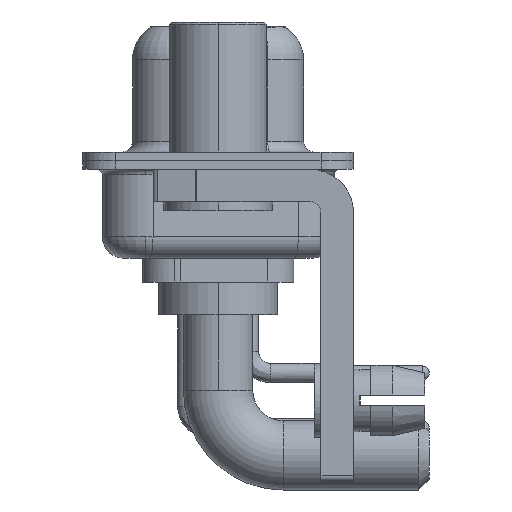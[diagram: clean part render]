
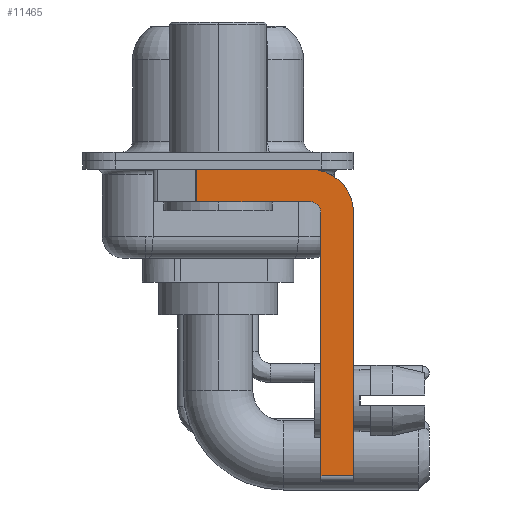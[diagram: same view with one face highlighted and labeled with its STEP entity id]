
A CAD part, left-side view. The second image highlights one B-rep face of the part: STEP entity #11465.
In plain terms, the highlighted planar face has unit normal (-1, 0, 0).
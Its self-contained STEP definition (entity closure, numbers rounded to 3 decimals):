
#335 = LINE ( 'NONE', #8071, #6720 ) ;
#677 = DIRECTION ( 'NONE',  ( -1., 0., 0. ) ) ;
#1410 = LINE ( 'NONE', #19088, #17224 ) ;
#1963 = CARTESIAN_POINT ( 'NONE',  ( -2.9, -4.25, -1.9 ) ) ;
#2416 = LINE ( 'NONE', #6575, #20677 ) ;
#2481 = VERTEX_POINT ( 'NONE', #11726 ) ;
#2768 = VERTEX_POINT ( 'NONE', #10321 ) ;
#3099 = DIRECTION ( 'NONE',  ( 0., 0., 1. ) ) ;
#3500 = LINE ( 'NONE', #6896, #24793 ) ;
#3735 = VERTEX_POINT ( 'NONE', #5189 ) ;
#4128 = EDGE_CURVE ( 'NONE', #4290, #12373, #3500, .T. ) ;
#4290 = VERTEX_POINT ( 'NONE', #1963 ) ;
#4563 = EDGE_CURVE ( 'NONE', #2481, #3735, #11192, .T. ) ;
#5189 = CARTESIAN_POINT ( 'NONE',  ( -2.9, -6.25, -2.4 ) ) ;
#6121 = ORIENTED_EDGE ( 'NONE', *, *, #11451, .F. ) ;
#6187 = DIRECTION ( 'NONE',  ( 0., 0., -1. ) ) ;
#6575 = CARTESIAN_POINT ( 'NONE',  ( -2.9, 0.978, -1.9 ) ) ;
#6720 = VECTOR ( 'NONE', #6187, 1000. ) ;
#6869 = DIRECTION ( 'NONE',  ( 1., 0., 0. ) ) ;
#6896 = CARTESIAN_POINT ( 'NONE',  ( -2.9, -4.25, -1.9 ) ) ;
#7363 = CARTESIAN_POINT ( 'NONE',  ( -2.9, 3., -0.4 ) ) ;
#7474 = CARTESIAN_POINT ( 'NONE',  ( -2.9, -4.75, -2.4 ) ) ;
#7487 = DIRECTION ( 'NONE',  ( 1., 0., 0. ) ) ;
#7610 = DIRECTION ( 'NONE',  ( 0., -1., 0. ) ) ;
#7772 = EDGE_CURVE ( 'NONE', #17053, #24008, #14337, .T. ) ;
#8071 = CARTESIAN_POINT ( 'NONE',  ( -2.9, -6.25, -2.4 ) ) ;
#8200 = VECTOR ( 'NONE', #12199, 1000. ) ;
#8413 = CARTESIAN_POINT ( 'NONE',  ( -2.9, -4.25, -2.4 ) ) ;
#8598 = DIRECTION ( 'NONE',  ( 0., 0., -1. ) ) ;
#8790 = ORIENTED_EDGE ( 'NONE', *, *, #18653, .F. ) ;
#9276 = AXIS2_PLACEMENT_3D ( 'NONE', #11174, #7487, #15063 ) ;
#9366 = ORIENTED_EDGE ( 'NONE', *, *, #7772, .T. ) ;
#9389 = LINE ( 'NONE', #7363, #24570 ) ;
#10321 = CARTESIAN_POINT ( 'NONE',  ( -2.9, 0.978, -0.4 ) ) ;
#10353 = ORIENTED_EDGE ( 'NONE', *, *, #20552, .F. ) ;
#11174 = CARTESIAN_POINT ( 'NONE',  ( -2.9, -4.25, -2.4 ) ) ;
#11192 = CIRCLE ( 'NONE', #16818, 2. ) ;
#11451 = EDGE_CURVE ( 'NONE', #2768, #2481, #9389, .T. ) ;
#11465 = ADVANCED_FACE ( 'NONE', ( #18844 ), #13289, .F. ) ;
#11726 = CARTESIAN_POINT ( 'NONE',  ( -2.9, -4.25, -0.4 ) ) ;
#12199 = DIRECTION ( 'NONE',  ( 0., -1., 0. ) ) ;
#12373 = VERTEX_POINT ( 'NONE', #19319 ) ;
#12914 = DIRECTION ( 'NONE',  ( 0., 0., 1. ) ) ;
#13289 = PLANE ( 'NONE',  #9276 ) ;
#14205 = CARTESIAN_POINT ( 'NONE',  ( -2.9, -4.25, -14.55 ) ) ;
#14337 = LINE ( 'NONE', #14205, #8200 ) ;
#14383 = CARTESIAN_POINT ( 'NONE',  ( -2.9, -6.25, -14.55 ) ) ;
#14894 = EDGE_CURVE ( 'NONE', #2768, #12373, #2416, .T. ) ;
#14950 = CARTESIAN_POINT ( 'NONE',  ( -2.9, -4.25, -2.4 ) ) ;
#15063 = DIRECTION ( 'NONE',  ( 0., 0., -1. ) ) ;
#15066 = ORIENTED_EDGE ( 'NONE', *, *, #4563, .F. ) ;
#15533 = CIRCLE ( 'NONE', #24396, 0.5 ) ;
#16152 = EDGE_LOOP ( 'NONE', ( #6121, #19538, #22775, #8790, #10353, #9366, #19533, #15066 ) ) ;
#16734 = DIRECTION ( 'NONE',  ( 0., 0., -1. ) ) ;
#16818 = AXIS2_PLACEMENT_3D ( 'NONE', #14950, #6869, #16734 ) ;
#17053 = VERTEX_POINT ( 'NONE', #18909 ) ;
#17224 = VECTOR ( 'NONE', #12914, 1000. ) ;
#18653 = EDGE_CURVE ( 'NONE', #19220, #4290, #15533, .T. ) ;
#18844 = FACE_OUTER_BOUND ( 'NONE', #16152, .T. ) ;
#18884 = DIRECTION ( 'NONE',  ( 0., 1., 0. ) ) ;
#18909 = CARTESIAN_POINT ( 'NONE',  ( -2.9, -4.75, -14.55 ) ) ;
#19088 = CARTESIAN_POINT ( 'NONE',  ( -2.9, -4.75, -14.8 ) ) ;
#19220 = VERTEX_POINT ( 'NONE', #7474 ) ;
#19319 = CARTESIAN_POINT ( 'NONE',  ( -2.9, 0.978, -1.9 ) ) ;
#19533 = ORIENTED_EDGE ( 'NONE', *, *, #19838, .F. ) ;
#19538 = ORIENTED_EDGE ( 'NONE', *, *, #14894, .T. ) ;
#19838 = EDGE_CURVE ( 'NONE', #3735, #24008, #335, .T. ) ;
#20552 = EDGE_CURVE ( 'NONE', #17053, #19220, #1410, .T. ) ;
#20677 = VECTOR ( 'NONE', #8598, 1000. ) ;
#22775 = ORIENTED_EDGE ( 'NONE', *, *, #4128, .F. ) ;
#24008 = VERTEX_POINT ( 'NONE', #14383 ) ;
#24396 = AXIS2_PLACEMENT_3D ( 'NONE', #8413, #677, #3099 ) ;
#24570 = VECTOR ( 'NONE', #7610, 1000. ) ;
#24793 = VECTOR ( 'NONE', #18884, 1000. ) ;
